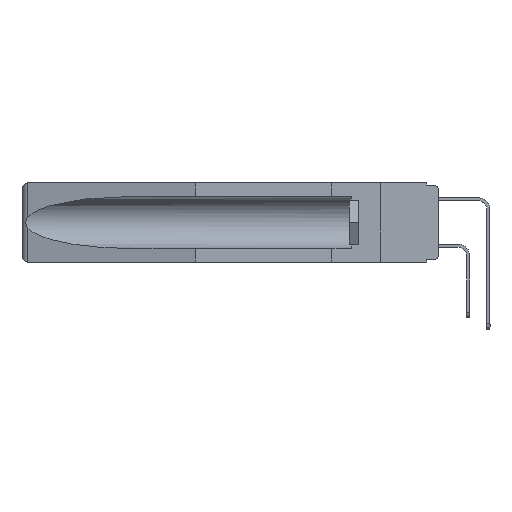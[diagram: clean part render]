
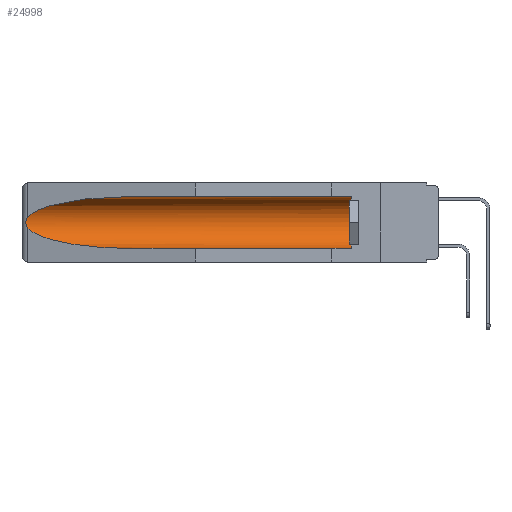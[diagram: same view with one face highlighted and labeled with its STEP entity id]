
A CAD part, left-side view. The second image highlights one B-rep face of the part: STEP entity #24998.
In plain terms, the highlighted cylindrical face has radius 2.857 mm (diameter 5.715 mm), a partial arc.
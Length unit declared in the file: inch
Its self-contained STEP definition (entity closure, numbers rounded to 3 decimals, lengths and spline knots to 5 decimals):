
#53 = EDGE_CURVE ( 'NONE', #5129, #8958, #16576, .T. ) ;
#695 = CARTESIAN_POINT ( 'NONE',  ( 0.21114, 1.30732, -0.284 ) ) ;
#1116 = ORIENTED_EDGE ( 'NONE', *, *, #53, .T. ) ;
#1357 = DIRECTION ( 'NONE',  ( 0., -1., 0. ) ) ;
#1362 = EDGE_CURVE ( 'NONE', #8958, #4733, #23949, .T. ) ;
#1432 = CARTESIAN_POINT ( 'NONE',  ( 0.25451, 1.48313, -0.09465 ) ) ;
#1471 = CARTESIAN_POINT ( 'NONE',  ( 0.155, 1.07973, -0.059 ) ) ;
#1822 = CARTESIAN_POINT ( 'NONE',  ( 0.155, -0.30754, -0.284 ) ) ;
#1847 = VERTEX_POINT ( 'NONE', #9642 ) ;
#2245 = DIRECTION ( 'NONE',  ( 0., 1., 0. ) ) ;
#2455 = DIRECTION ( 'NONE',  ( 0., 0., 1. ) ) ;
#3001 = CARTESIAN_POINT ( 'NONE',  ( 0.155, 0.126, -0.284 ) ) ;
#3138 = CARTESIAN_POINT ( 'NONE',  ( 0.155, 0.126, -0.059 ) ) ;
#3142 = VECTOR ( 'NONE', #23671, 39.37008 ) ;
#3358 = AXIS2_PLACEMENT_3D ( 'NONE', #13196, #22351, #2455 ) ;
#3711 = CARTESIAN_POINT ( 'NONE',  ( 0.26537, 1.52718, -0.14972 ) ) ;
#4021 = CARTESIAN_POINT ( 'NONE',  ( 0.26655, 1.53094, -0.18657 ) ) ;
#4300 = CARTESIAN_POINT ( 'NONE',  ( 0.26537, 1.52718, -0.19328 ) ) ;
#4341 = CARTESIAN_POINT ( 'NONE',  ( 0.155, -0.30754, -0.059 ) ) ;
#4435 = CARTESIAN_POINT ( 'NONE',  ( 0.2675, 1.53308, -0.17534 ) ) ;
#4629 =( BOUNDED_CURVE ( )  B_SPLINE_CURVE ( 3, ( #27467, #10301, #1432, #3711 ),
 .UNSPECIFIED., .F., .F. ) 
 B_SPLINE_CURVE_WITH_KNOTS ( ( 4, 4 ),
 ( 4.71239, 6.08839 ),
 .UNSPECIFIED. ) 
 CURVE ( )  GEOMETRIC_REPRESENTATION_ITEM ( )  RATIONAL_B_SPLINE_CURVE ( ( 1., 0.848, 0.848, 1. ) ) 
 REPRESENTATION_ITEM ( '' )  );
#4733 = VERTEX_POINT ( 'NONE', #1471 ) ;
#5129 = VERTEX_POINT ( 'NONE', #3001 ) ;
#5487 = CARTESIAN_POINT ( 'NONE',  ( 0.155, 0.126, -0.1715 ) ) ;
#8046 = EDGE_LOOP ( 'NONE', ( #14226, #21139, #12338, #25334, #1116, #9606 ) ) ;
#8396 = LINE ( 'NONE', #1822, #24822 ) ;
#8958 = VERTEX_POINT ( 'NONE', #3138 ) ;
#9182 = CARTESIAN_POINT ( 'NONE',  ( 0.26537, 1.52718, -0.19328 ) ) ;
#9606 = ORIENTED_EDGE ( 'NONE', *, *, #1362, .T. ) ;
#9642 = CARTESIAN_POINT ( 'NONE',  ( 0.26537, 1.52718, -0.14972 ) ) ;
#10301 = CARTESIAN_POINT ( 'NONE',  ( 0.21114, 1.30732, -0.059 ) ) ;
#10597 = VERTEX_POINT ( 'NONE', #26087 ) ;
#12338 = ORIENTED_EDGE ( 'NONE', *, *, #25640, .T. ) ;
#13196 = CARTESIAN_POINT ( 'NONE',  ( 0.155, -0.30754, -0.1715 ) ) ;
#13315 = CARTESIAN_POINT ( 'NONE',  ( 0.26597, 1.52961, -0.15275 ) ) ;
#13750 = EDGE_CURVE ( 'NONE', #1847, #16758, #18646, .T. ) ;
#14226 = ORIENTED_EDGE ( 'NONE', *, *, #21321, .T. ) ;
#14917 = CARTESIAN_POINT ( 'NONE',  ( 0.26537, 1.52718, -0.14972 ) ) ;
#15884 = CARTESIAN_POINT ( 'NONE',  ( 0.25451, 1.48313, -0.24835 ) ) ;
#16576 = CIRCLE ( 'NONE', #20230, 0.1125 ) ;
#16758 = VERTEX_POINT ( 'NONE', #9182 ) ;
#17070 = CARTESIAN_POINT ( 'NONE',  ( 0.2673, 1.5327, -0.16383 ) ) ;
#18431 = CARTESIAN_POINT ( 'NONE',  ( 0.155, 1.07973, -0.284 ) ) ;
#18646 = B_SPLINE_CURVE_WITH_KNOTS ( 'NONE', 3,
 ( #14917, #13315, #23631, #17070, #22055, #4435, #21919, #4021, #25783, #4300 ),
 .UNSPECIFIED., .F., .F.,
 ( 4, 2, 2, 2, 4 ),
 ( 0., 0.00029, 0.00058, 0.00087, 0.00117 ),
 .UNSPECIFIED. ) ;
#19921 = EDGE_CURVE ( 'NONE', #5129, #10597, #8396, .T. ) ;
#20230 = AXIS2_PLACEMENT_3D ( 'NONE', #5487, #1357, #22945 ) ;
#21139 = ORIENTED_EDGE ( 'NONE', *, *, #13750, .T. ) ;
#21321 = EDGE_CURVE ( 'NONE', #4733, #1847, #4629, .T. ) ;
#21919 = CARTESIAN_POINT ( 'NONE',  ( 0.2673, 1.53269, -0.17917 ) ) ;
#22055 = CARTESIAN_POINT ( 'NONE',  ( 0.2675, 1.53308, -0.16763 ) ) ;
#22351 = DIRECTION ( 'NONE',  ( 0., 1., 0. ) ) ;
#22945 = DIRECTION ( 'NONE',  ( 0., 0., 1. ) ) ;
#23631 = CARTESIAN_POINT ( 'NONE',  ( 0.26654, 1.53092, -0.15636 ) ) ;
#23671 = DIRECTION ( 'NONE',  ( 0., 1., 0. ) ) ;
#23949 = LINE ( 'NONE', #4341, #3142 ) ;
#24822 = VECTOR ( 'NONE', #2245, 39.37008 ) ;
#24998 = ADVANCED_FACE ( 'NONE', ( #26643 ), #26220, .F. ) ;
#25334 = ORIENTED_EDGE ( 'NONE', *, *, #19921, .F. ) ;
#25640 = EDGE_CURVE ( 'NONE', #16758, #10597, #28197, .T. ) ;
#25783 = CARTESIAN_POINT ( 'NONE',  ( 0.26597, 1.5296, -0.19026 ) ) ;
#26087 = CARTESIAN_POINT ( 'NONE',  ( 0.155, 1.07973, -0.284 ) ) ;
#26220 = CYLINDRICAL_SURFACE ( 'NONE', #3358, 0.1125 ) ;
#26643 = FACE_OUTER_BOUND ( 'NONE', #8046, .T. ) ;
#26881 = CARTESIAN_POINT ( 'NONE',  ( 0.26537, 1.52718, -0.19328 ) ) ;
#27467 = CARTESIAN_POINT ( 'NONE',  ( 0.155, 1.07973, -0.059 ) ) ;
#28197 =( BOUNDED_CURVE ( )  B_SPLINE_CURVE ( 3, ( #26881, #15884, #695, #18431 ),
 .UNSPECIFIED., .F., .F. ) 
 B_SPLINE_CURVE_WITH_KNOTS ( ( 4, 4 ),
 ( 0.1948, 1.5708 ),
 .UNSPECIFIED. ) 
 CURVE ( )  GEOMETRIC_REPRESENTATION_ITEM ( )  RATIONAL_B_SPLINE_CURVE ( ( 1., 0.848, 0.848, 1. ) ) 
 REPRESENTATION_ITEM ( '' )  );
